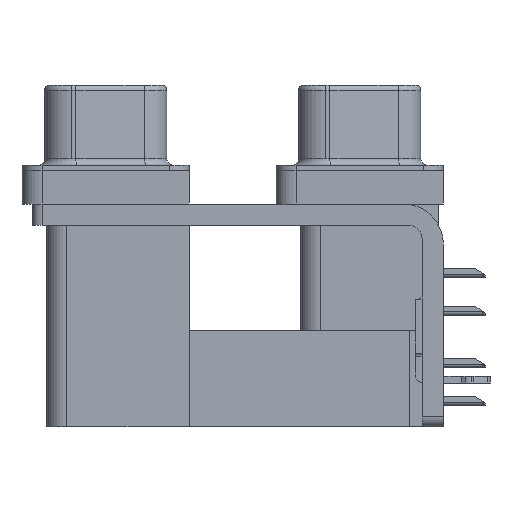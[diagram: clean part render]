
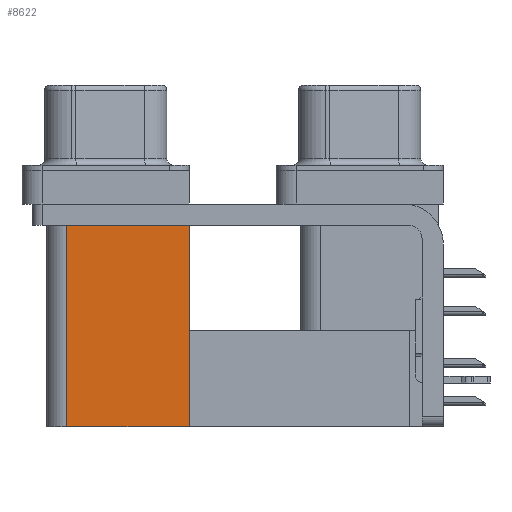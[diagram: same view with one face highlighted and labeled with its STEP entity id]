
A CAD part, left-side view. The second image highlights one B-rep face of the part: STEP entity #8622.
In plain terms, the highlighted planar face has unit normal (-1, 0, 0).
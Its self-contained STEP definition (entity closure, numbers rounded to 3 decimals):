
#487 = LINE ( 'NONE', #15300, #7194 ) ;
#1234 = AXIS2_PLACEMENT_3D ( 'NONE', #18970, #23802, #28494 ) ;
#1982 = ORIENTED_EDGE ( 'NONE', *, *, #28413, .F. ) ;
#2073 = CARTESIAN_POINT ( 'NONE',  ( 3.765, 12.775, -2.5 ) ) ;
#3659 = VECTOR ( 'NONE', #11598, 1000. ) ;
#4054 = DIRECTION ( 'NONE',  ( 0., 0., 1. ) ) ;
#4923 = FACE_OUTER_BOUND ( 'NONE', #7052, .T. ) ;
#6371 = VERTEX_POINT ( 'NONE', #6699 ) ;
#6699 = CARTESIAN_POINT ( 'NONE',  ( 3.765, 12.775, -19.2 ) ) ;
#7052 = EDGE_LOOP ( 'NONE', ( #30037, #18024, #1982, #16361 ) ) ;
#7194 = VECTOR ( 'NONE', #12957, 1000. ) ;
#8246 = LINE ( 'NONE', #27419, #30240 ) ;
#8377 = CARTESIAN_POINT ( 'NONE',  ( 3.765, 21.975, -2.5 ) ) ;
#8622 = ADVANCED_FACE ( 'NONE', ( #4923 ), #17240, .F. ) ;
#8761 = VECTOR ( 'NONE', #4054, 1000. ) ;
#10992 = EDGE_CURVE ( 'NONE', #13451, #22343, #30169, .T. ) ;
#11089 = CARTESIAN_POINT ( 'NONE',  ( 3.765, 12.775, -19.2 ) ) ;
#11598 = DIRECTION ( 'NONE',  ( 0., 1., 0. ) ) ;
#12957 = DIRECTION ( 'NONE',  ( 0., 0., 1. ) ) ;
#13432 = LINE ( 'NONE', #11089, #8761 ) ;
#13451 = VERTEX_POINT ( 'NONE', #15985 ) ;
#14186 = EDGE_CURVE ( 'NONE', #22390, #22343, #487, .T. ) ;
#14937 = CARTESIAN_POINT ( 'NONE',  ( 3.765, 21.975, -19.2 ) ) ;
#15300 = CARTESIAN_POINT ( 'NONE',  ( 3.765, 21.975, -19.2 ) ) ;
#15985 = CARTESIAN_POINT ( 'NONE',  ( 3.765, 12.775, -2.5 ) ) ;
#16361 = ORIENTED_EDGE ( 'NONE', *, *, #25558, .T. ) ;
#17240 = PLANE ( 'NONE',  #1234 ) ;
#18024 = ORIENTED_EDGE ( 'NONE', *, *, #14186, .F. ) ;
#18970 = CARTESIAN_POINT ( 'NONE',  ( 3.765, 12.775, -19.2 ) ) ;
#20702 = DIRECTION ( 'NONE',  ( 0., 1., 0. ) ) ;
#22343 = VERTEX_POINT ( 'NONE', #8377 ) ;
#22390 = VERTEX_POINT ( 'NONE', #14937 ) ;
#23802 = DIRECTION ( 'NONE',  ( 1., 0., 0. ) ) ;
#25558 = EDGE_CURVE ( 'NONE', #6371, #13451, #13432, .T. ) ;
#27419 = CARTESIAN_POINT ( 'NONE',  ( 3.765, 12.775, -19.2 ) ) ;
#28413 = EDGE_CURVE ( 'NONE', #6371, #22390, #8246, .T. ) ;
#28494 = DIRECTION ( 'NONE',  ( 0., 0., -1. ) ) ;
#30037 = ORIENTED_EDGE ( 'NONE', *, *, #10992, .T. ) ;
#30169 = LINE ( 'NONE', #2073, #3659 ) ;
#30240 = VECTOR ( 'NONE', #20702, 1000. ) ;
